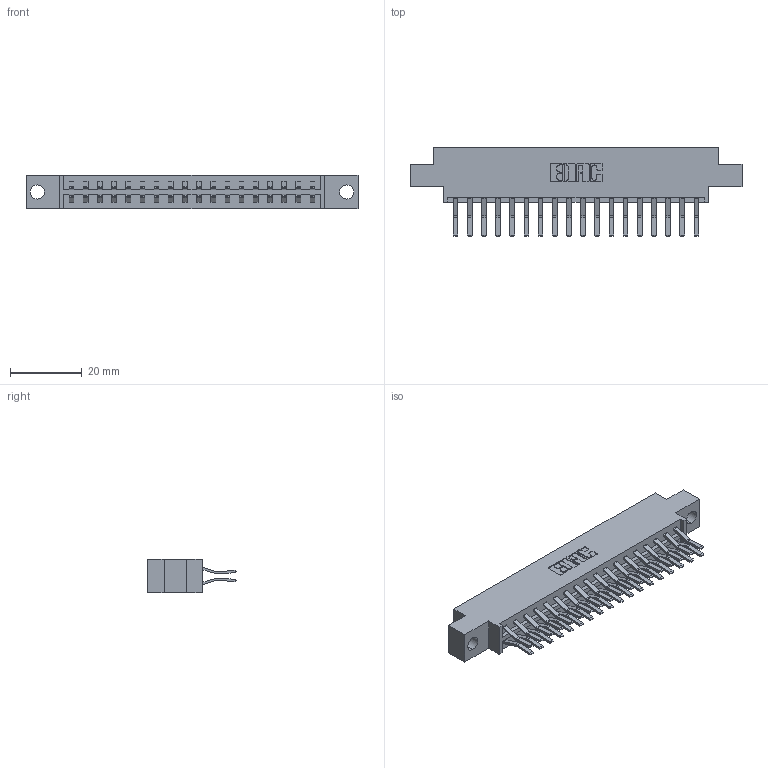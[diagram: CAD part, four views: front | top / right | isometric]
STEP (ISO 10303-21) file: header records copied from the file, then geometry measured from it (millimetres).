
FILE_DESCRIPTION (( 'STEP AP203' ), '1' );
FILE_NAME ('833-036-560-804.STEP', '2020-06-03T04:28:08', ( '' ), ( '' ), 'SwSTEP 2.0', 'SolidWorks 2020', '' );
FILE_SCHEMA (( 'CONFIG_CONTROL_DESIGN' ));
Length unit declared in the file: inch
Products named in the file (3): 833-036-560-804; 345-292-001_560 Tail; 833 Part_Offset - .156 Dia - TH
Assembly tree (37 placements, depth 2):
  833-036-560-804
    833 Part_Offset - .156 Dia - TH
    345-292-001_560 Tail  x36
Bounding box: 92.86 x 24.78 x 9.4 mm (x, y, z)
Volume: 9176.6 mm3; surface area: 11284.5 mm2
Topology: 37 solids, 37 shells, 2062 faces, 6119 edges, 4030 vertices
Faces by surface type: plane 1370, cylinder 692
Entity records: 14907 total; most frequent: CARTESIAN_POINT 2502, ORIENTED_EDGE 2438, DIRECTION 2183, EDGE_CURVE 1219, LINE 1087, VECTOR 1087, VERTEX_POINT 810, AXIS2_PLACEMENT_3D 548
